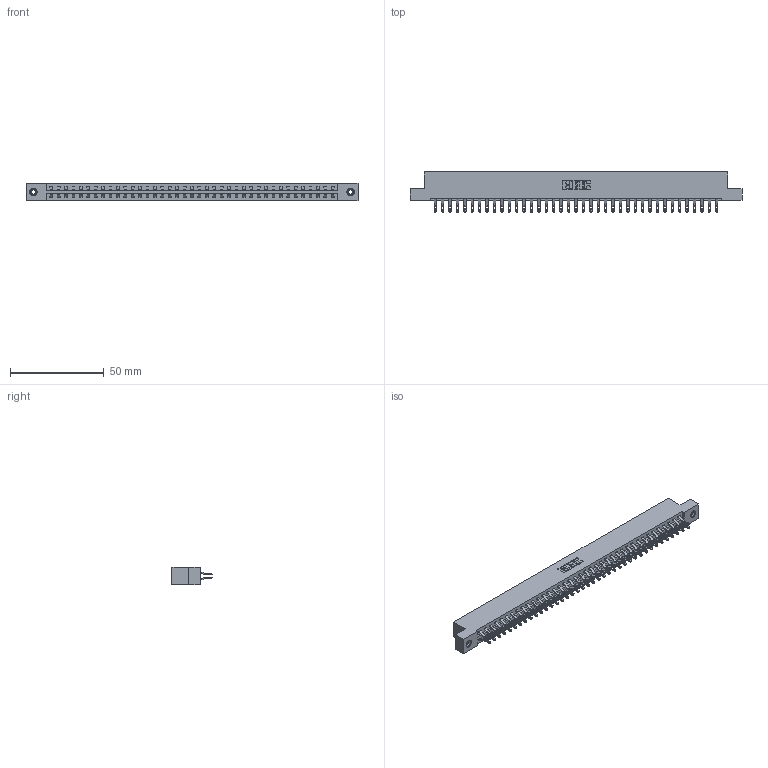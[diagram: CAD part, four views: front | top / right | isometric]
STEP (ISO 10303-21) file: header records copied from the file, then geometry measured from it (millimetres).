
FILE_DESCRIPTION (( 'STEP AP203' ), '1' );
FILE_NAME ('337-078-555-208.STEP', '2018-08-12T16:29:10', ( '' ), ( '' ), 'SwSTEP 2.0', 'SolidWorks 2016', '' );
FILE_SCHEMA (( 'CONFIG_CONTROL_DESIGN' ));
Length unit declared in the file: inch
Products named in the file (4): 337-078-555-208; 337 Part_Flush Mounting Lugs - 0.156 Dia-TI; 345-292-001_555 Tail; 345-250-001_345-250-003-102
Assembly tree (81 placements, depth 2):
  337-078-555-208
    337 Part_Flush Mounting Lugs - 0.156 Dia-TI
    345-292-001_555 Tail  x78
    345-250-001_345-250-003-102  x2
Bounding box: 177.55 x 21.47 x 9.4 mm (x, y, z)
Volume: 18891 mm3; surface area: 22203.7 mm2
Topology: 81 solids, 81 shells, 4854 faces, 15189 edges, 10118 vertices
Faces by surface type: plane 2910, cylinder 1928, cone 12, torus 4
Entity records: 32138 total; most frequent: CARTESIAN_POINT 5431, ORIENTED_EDGE 5330, DIRECTION 4627, EDGE_CURVE 2665, LINE 2497, VECTOR 2497, VERTEX_POINT 1772, AXIS2_PLACEMENT_3D 1065
